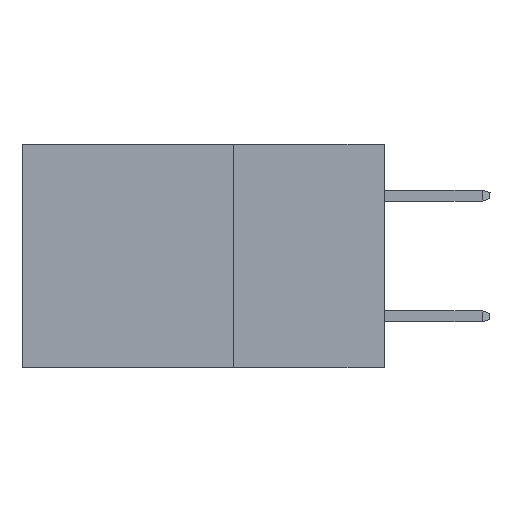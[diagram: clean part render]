
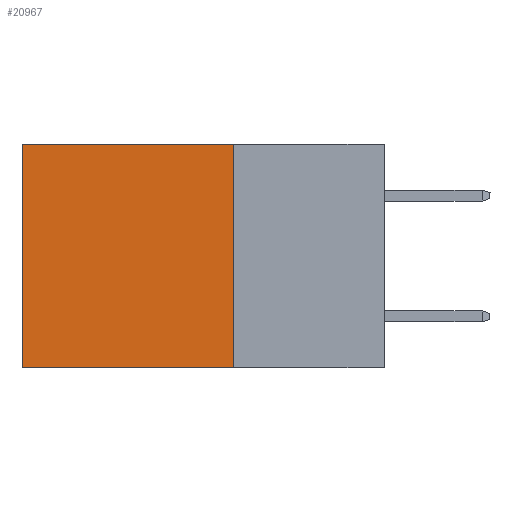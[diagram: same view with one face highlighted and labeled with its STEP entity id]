
A CAD part, left-side view. The second image highlights one B-rep face of the part: STEP entity #20967.
In plain terms, the highlighted planar face has unit normal (-1, 0, 0).
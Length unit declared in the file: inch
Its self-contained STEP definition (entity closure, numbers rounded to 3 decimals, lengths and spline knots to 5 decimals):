
#1551 = DIRECTION ( 'NONE',  ( 0., 0., -1. ) ) ;
#1848 = CARTESIAN_POINT ( 'NONE',  ( 0.298, 0.25, -0.37 ) ) ;
#2656 = PLANE ( 'NONE',  #3077 ) ;
#2704 = VECTOR ( 'NONE', #4185, 39.37008 ) ;
#2756 = VECTOR ( 'NONE', #14231, 39.37008 ) ;
#2934 = EDGE_CURVE ( 'NONE', #10821, #10737, #14374, .T. ) ;
#2957 = LINE ( 'NONE', #22054, #5764 ) ;
#2990 = LINE ( 'NONE', #10389, #12709 ) ;
#3077 = AXIS2_PLACEMENT_3D ( 'NONE', #13120, #14898, #20320 ) ;
#3709 = ORIENTED_EDGE ( 'NONE', *, *, #22399, .F. ) ;
#3861 = EDGE_CURVE ( 'NONE', #10737, #9802, #2957, .T. ) ;
#4185 = DIRECTION ( 'NONE',  ( 0., 1., 0. ) ) ;
#4756 = ORIENTED_EDGE ( 'NONE', *, *, #17437, .F. ) ;
#5764 = VECTOR ( 'NONE', #1551, 39.37008 ) ;
#6381 = ORIENTED_EDGE ( 'NONE', *, *, #2934, .T. ) ;
#7844 = ORIENTED_EDGE ( 'NONE', *, *, #3861, .T. ) ;
#8024 = LINE ( 'NONE', #1848, #2756 ) ;
#9802 = VERTEX_POINT ( 'NONE', #13637 ) ;
#10088 = FACE_OUTER_BOUND ( 'NONE', #17003, .T. ) ;
#10389 = CARTESIAN_POINT ( 'NONE',  ( 0.298, 0.25, 0. ) ) ;
#10737 = VERTEX_POINT ( 'NONE', #11264 ) ;
#10821 = VERTEX_POINT ( 'NONE', #22834 ) ;
#11264 = CARTESIAN_POINT ( 'NONE',  ( 0.298, 0.6, 0. ) ) ;
#12709 = VECTOR ( 'NONE', #22677, 39.37008 ) ;
#13120 = CARTESIAN_POINT ( 'NONE',  ( 0.298, 0.25, 0. ) ) ;
#13500 = CARTESIAN_POINT ( 'NONE',  ( 0.298, 0.25, -0.37 ) ) ;
#13637 = CARTESIAN_POINT ( 'NONE',  ( 0.298, 0.6, -0.37 ) ) ;
#14231 = DIRECTION ( 'NONE',  ( 0., 1., 0. ) ) ;
#14374 = LINE ( 'NONE', #21983, #2704 ) ;
#14898 = DIRECTION ( 'NONE',  ( 1., 0., 0. ) ) ;
#17003 = EDGE_LOOP ( 'NONE', ( #7844, #4756, #3709, #6381 ) ) ;
#17437 = EDGE_CURVE ( 'NONE', #21049, #9802, #8024, .T. ) ;
#20320 = DIRECTION ( 'NONE',  ( 0., 0., -1. ) ) ;
#20967 = ADVANCED_FACE ( 'NONE', ( #10088 ), #2656, .F. ) ;
#21049 = VERTEX_POINT ( 'NONE', #13500 ) ;
#21983 = CARTESIAN_POINT ( 'NONE',  ( 0.298, 0.25, 0. ) ) ;
#22054 = CARTESIAN_POINT ( 'NONE',  ( 0.298, 0.6, 0. ) ) ;
#22399 = EDGE_CURVE ( 'NONE', #10821, #21049, #2990, .T. ) ;
#22677 = DIRECTION ( 'NONE',  ( 0., 0., -1. ) ) ;
#22834 = CARTESIAN_POINT ( 'NONE',  ( 0.298, 0.25, 0. ) ) ;
